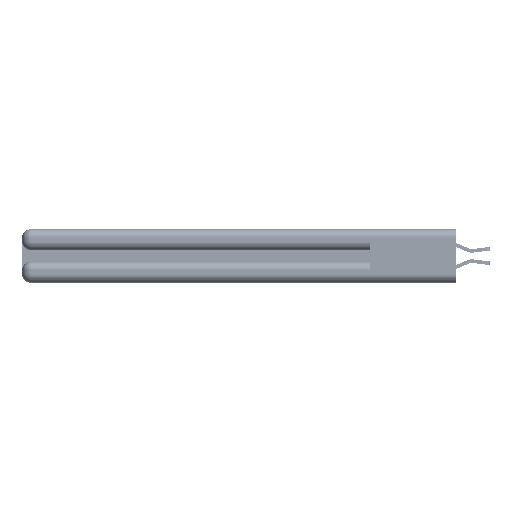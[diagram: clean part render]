
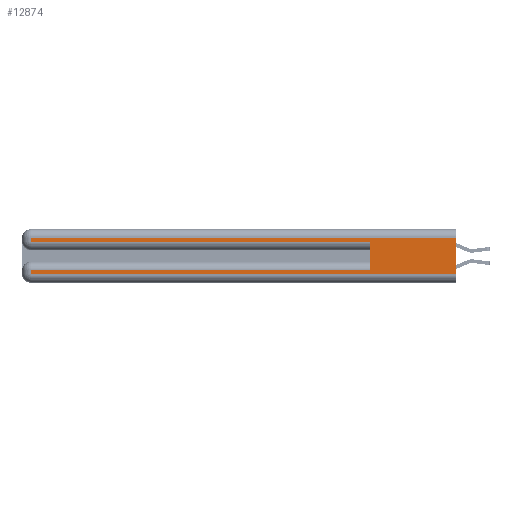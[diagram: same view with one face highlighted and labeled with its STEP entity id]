
A CAD part, left-side view. The second image highlights one B-rep face of the part: STEP entity #12874.
In plain terms, the highlighted planar face has unit normal (-1, 0, 0).
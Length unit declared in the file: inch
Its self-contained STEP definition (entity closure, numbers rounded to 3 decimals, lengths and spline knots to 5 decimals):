
#182 = EDGE_CURVE ( 'NONE', #34734, #1601, #43385, .T. ) ;
#1189 = CARTESIAN_POINT ( 'NONE',  ( 0., 0.6, 0.085 ) ) ;
#1527 = CARTESIAN_POINT ( 'NONE',  ( 0., 2.94, 0.37 ) ) ;
#1601 = VERTEX_POINT ( 'NONE', #40817 ) ;
#1840 = VECTOR ( 'NONE', #3800, 39.37008 ) ;
#2699 = FACE_OUTER_BOUND ( 'NONE', #19599, .T. ) ;
#3800 = DIRECTION ( 'NONE',  ( 0., 1., 0. ) ) ;
#4053 = LINE ( 'NONE', #8616, #10438 ) ;
#6402 = LINE ( 'NONE', #19338, #40740 ) ;
#6465 = ORIENTED_EDGE ( 'NONE', *, *, #33455, .T. ) ;
#8207 = DIRECTION ( 'NONE',  ( 0., -1., 0. ) ) ;
#8616 = CARTESIAN_POINT ( 'NONE',  ( 0., 0., 0.285 ) ) ;
#10438 = VECTOR ( 'NONE', #8207, 39.37008 ) ;
#11994 = VERTEX_POINT ( 'NONE', #51562 ) ;
#12874 = ADVANCED_FACE ( 'NONE', ( #2699 ), #17233, .F. ) ;
#13997 = CARTESIAN_POINT ( 'NONE',  ( 0., 0., 0.085 ) ) ;
#14230 = ORIENTED_EDGE ( 'NONE', *, *, #42002, .T. ) ;
#15309 = DIRECTION ( 'NONE',  ( 0., 0., -1. ) ) ;
#15409 = LINE ( 'NONE', #43975, #1840 ) ;
#17233 = PLANE ( 'NONE',  #39502 ) ;
#18951 = VERTEX_POINT ( 'NONE', #20288 ) ;
#19338 = CARTESIAN_POINT ( 'NONE',  ( 0., 2.94, 0.37 ) ) ;
#19345 = ORIENTED_EDGE ( 'NONE', *, *, #45361, .T. ) ;
#19473 = LINE ( 'NONE', #38041, #40385 ) ;
#19599 = EDGE_LOOP ( 'NONE', ( #23742, #21779, #29522, #19345, #20082, #43144, #6465, #14230 ) ) ;
#20082 = ORIENTED_EDGE ( 'NONE', *, *, #182, .F. ) ;
#20288 = CARTESIAN_POINT ( 'NONE',  ( 0., 0., 0.31 ) ) ;
#20716 = DIRECTION ( 'NONE',  ( 0., 0., 1. ) ) ;
#21237 = EDGE_CURVE ( 'NONE', #18951, #11994, #15409, .T. ) ;
#21513 = EDGE_CURVE ( 'NONE', #34734, #31135, #47440, .T. ) ;
#21779 = ORIENTED_EDGE ( 'NONE', *, *, #21237, .T. ) ;
#22920 = CARTESIAN_POINT ( 'NONE',  ( 0., 0., 0.06 ) ) ;
#23742 = ORIENTED_EDGE ( 'NONE', *, *, #50962, .F. ) ;
#25369 = EDGE_CURVE ( 'NONE', #11994, #46557, #6402, .T. ) ;
#26240 = CARTESIAN_POINT ( 'NONE',  ( 0., 2.94, 0.285 ) ) ;
#26309 = DIRECTION ( 'NONE',  ( 1., 0., 0. ) ) ;
#27431 = DIRECTION ( 'NONE',  ( 0., -1., 0. ) ) ;
#27581 = DIRECTION ( 'NONE',  ( 0., 1., 0. ) ) ;
#29522 = ORIENTED_EDGE ( 'NONE', *, *, #25369, .T. ) ;
#31135 = VERTEX_POINT ( 'NONE', #32263 ) ;
#31646 = VECTOR ( 'NONE', #20716, 39.37008 ) ;
#32263 = CARTESIAN_POINT ( 'NONE',  ( 0., 2.94, 0.085 ) ) ;
#32367 = LINE ( 'NONE', #22920, #54448 ) ;
#33455 = EDGE_CURVE ( 'NONE', #31135, #57949, #44251, .T. ) ;
#33987 = CARTESIAN_POINT ( 'NONE',  ( 0., 0.6, 0.145 ) ) ;
#34295 = VECTOR ( 'NONE', #27581, 39.37008 ) ;
#34734 = VERTEX_POINT ( 'NONE', #1189 ) ;
#37082 = DIRECTION ( 'NONE',  ( 0., 0., -1. ) ) ;
#38041 = CARTESIAN_POINT ( 'NONE',  ( 0., 0., 0.37 ) ) ;
#39502 = AXIS2_PLACEMENT_3D ( 'NONE', #52790, #26309, #57228 ) ;
#40385 = VECTOR ( 'NONE', #51358, 39.37008 ) ;
#40740 = VECTOR ( 'NONE', #37082, 39.37008 ) ;
#40817 = CARTESIAN_POINT ( 'NONE',  ( 0., 0.6, 0.285 ) ) ;
#42002 = EDGE_CURVE ( 'NONE', #57949, #54908, #32367, .T. ) ;
#43144 = ORIENTED_EDGE ( 'NONE', *, *, #21513, .T. ) ;
#43385 = LINE ( 'NONE', #33987, #31646 ) ;
#43975 = CARTESIAN_POINT ( 'NONE',  ( 0., 0., 0.31 ) ) ;
#44251 = LINE ( 'NONE', #1527, #54597 ) ;
#45361 = EDGE_CURVE ( 'NONE', #46557, #1601, #4053, .T. ) ;
#46557 = VERTEX_POINT ( 'NONE', #26240 ) ;
#46826 = CARTESIAN_POINT ( 'NONE',  ( 0., 2.94, 0.06 ) ) ;
#47440 = LINE ( 'NONE', #13997, #34295 ) ;
#48690 = CARTESIAN_POINT ( 'NONE',  ( 0., 0., 0.06 ) ) ;
#50962 = EDGE_CURVE ( 'NONE', #18951, #54908, #19473, .T. ) ;
#51358 = DIRECTION ( 'NONE',  ( 0., 0., -1. ) ) ;
#51562 = CARTESIAN_POINT ( 'NONE',  ( 0., 2.94, 0.31 ) ) ;
#52790 = CARTESIAN_POINT ( 'NONE',  ( 0., 0., 0.37 ) ) ;
#54448 = VECTOR ( 'NONE', #27431, 39.37008 ) ;
#54597 = VECTOR ( 'NONE', #15309, 39.37008 ) ;
#54908 = VERTEX_POINT ( 'NONE', #48690 ) ;
#57228 = DIRECTION ( 'NONE',  ( 0., 0., -1. ) ) ;
#57949 = VERTEX_POINT ( 'NONE', #46826 ) ;
